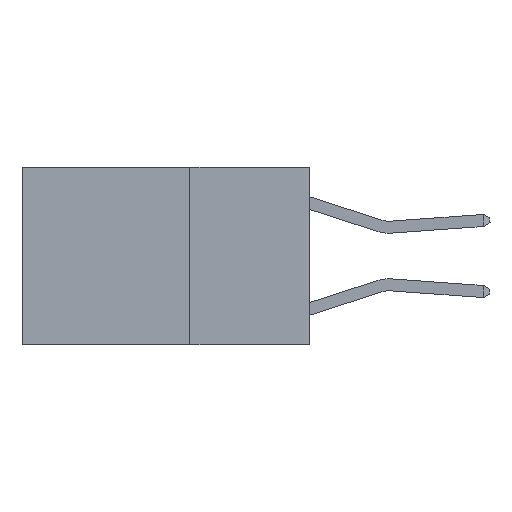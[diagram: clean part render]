
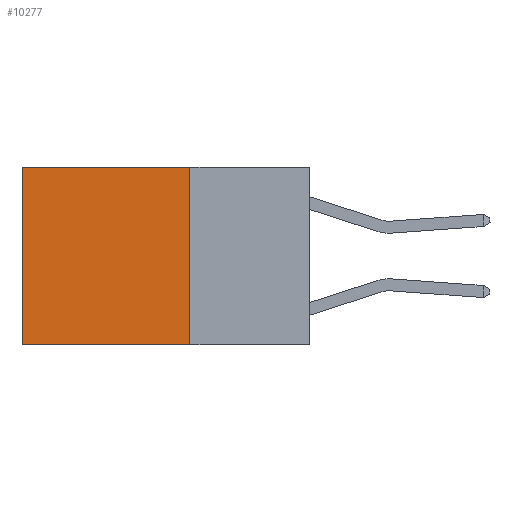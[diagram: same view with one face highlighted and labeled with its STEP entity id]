
A CAD part, left-side view. The second image highlights one B-rep face of the part: STEP entity #10277.
In plain terms, the highlighted planar face has unit normal (-1, 0, 0).
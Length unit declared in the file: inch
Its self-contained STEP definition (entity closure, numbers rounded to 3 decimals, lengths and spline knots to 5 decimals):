
#977 = EDGE_CURVE ( 'NONE', #1187, #5237, #3804, .T. ) ;
#1187 = VERTEX_POINT ( 'NONE', #2755 ) ;
#1480 = VECTOR ( 'NONE', #3637, 39.37008 ) ;
#1777 = CARTESIAN_POINT ( 'NONE',  ( 0.2625, 0.25, 0. ) ) ;
#2266 = CARTESIAN_POINT ( 'NONE',  ( 0.2625, 0.25, 0. ) ) ;
#2365 = CARTESIAN_POINT ( 'NONE',  ( 0.2625, 0.25, -0.37 ) ) ;
#2625 = CARTESIAN_POINT ( 'NONE',  ( 0.2625, 0.25, 0. ) ) ;
#2704 = DIRECTION ( 'NONE',  ( 0., 1., 0. ) ) ;
#2755 = CARTESIAN_POINT ( 'NONE',  ( 0.2625, 0.25, -0.37 ) ) ;
#3005 = ORIENTED_EDGE ( 'NONE', *, *, #3793, .F. ) ;
#3016 = CARTESIAN_POINT ( 'NONE',  ( 0.2625, 0.6, -0.37 ) ) ;
#3299 = DIRECTION ( 'NONE',  ( 0., 1., 0. ) ) ;
#3574 = DIRECTION ( 'NONE',  ( 1., 0., 0. ) ) ;
#3637 = DIRECTION ( 'NONE',  ( 0., 0., -1. ) ) ;
#3672 = LINE ( 'NONE', #8925, #1480 ) ;
#3793 = EDGE_CURVE ( 'NONE', #5275, #1187, #4713, .T. ) ;
#3804 = LINE ( 'NONE', #2365, #8284 ) ;
#3954 = VERTEX_POINT ( 'NONE', #9437 ) ;
#4188 = EDGE_CURVE ( 'NONE', #3954, #5237, #3672, .T. ) ;
#4603 = LINE ( 'NONE', #1777, #6403 ) ;
#4713 = LINE ( 'NONE', #2266, #5263 ) ;
#5237 = VERTEX_POINT ( 'NONE', #3016 ) ;
#5263 = VECTOR ( 'NONE', #8544, 39.37008 ) ;
#5275 = VERTEX_POINT ( 'NONE', #10047 ) ;
#6403 = VECTOR ( 'NONE', #2704, 39.37008 ) ;
#7672 = ORIENTED_EDGE ( 'NONE', *, *, #977, .F. ) ;
#7953 = ORIENTED_EDGE ( 'NONE', *, *, #4188, .T. ) ;
#8284 = VECTOR ( 'NONE', #3299, 39.37008 ) ;
#8544 = DIRECTION ( 'NONE',  ( 0., 0., -1. ) ) ;
#8865 = PLANE ( 'NONE',  #9404 ) ;
#8925 = CARTESIAN_POINT ( 'NONE',  ( 0.2625, 0.6, 0. ) ) ;
#9319 = EDGE_LOOP ( 'NONE', ( #7953, #7672, #3005, #10574 ) ) ;
#9404 = AXIS2_PLACEMENT_3D ( 'NONE', #2625, #3574, #9658 ) ;
#9437 = CARTESIAN_POINT ( 'NONE',  ( 0.2625, 0.6, 0. ) ) ;
#9658 = DIRECTION ( 'NONE',  ( 0., 0., -1. ) ) ;
#10047 = CARTESIAN_POINT ( 'NONE',  ( 0.2625, 0.25, 0. ) ) ;
#10277 = ADVANCED_FACE ( 'NONE', ( #11058 ), #8865, .F. ) ;
#10341 = EDGE_CURVE ( 'NONE', #5275, #3954, #4603, .T. ) ;
#10574 = ORIENTED_EDGE ( 'NONE', *, *, #10341, .T. ) ;
#11058 = FACE_OUTER_BOUND ( 'NONE', #9319, .T. ) ;
